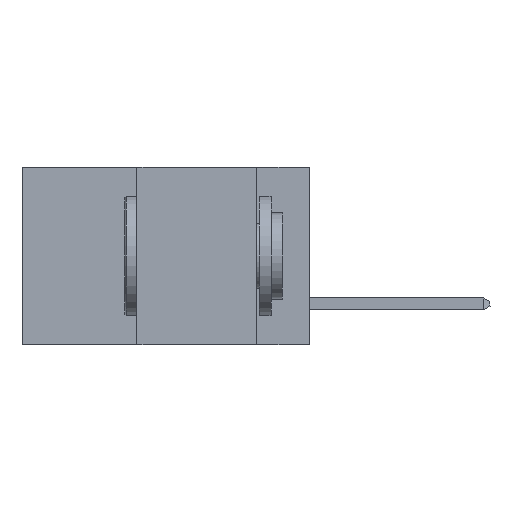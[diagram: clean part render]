
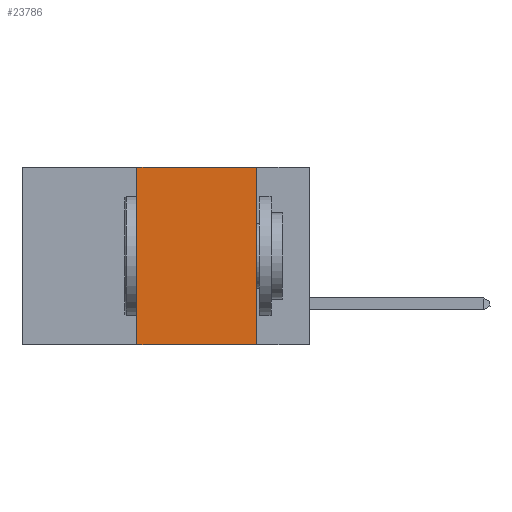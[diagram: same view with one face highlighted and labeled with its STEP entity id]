
A CAD part, left-side view. The second image highlights one B-rep face of the part: STEP entity #23786.
In plain terms, the highlighted planar face has unit normal (-1, 0, 0).
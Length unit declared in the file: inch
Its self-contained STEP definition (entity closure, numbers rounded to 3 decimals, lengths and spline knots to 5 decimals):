
#827 = DIRECTION ( 'NONE',  ( 0., -1., 0. ) ) ;
#1210 = CARTESIAN_POINT ( 'NONE',  ( 0., 0.36, -0.37 ) ) ;
#1501 = VECTOR ( 'NONE', #12696, 39.37008 ) ;
#2147 = VECTOR ( 'NONE', #4223, 39.37008 ) ;
#4177 = VERTEX_POINT ( 'NONE', #1210 ) ;
#4223 = DIRECTION ( 'NONE',  ( 0., 0., 1. ) ) ;
#4787 = CARTESIAN_POINT ( 'NONE',  ( 0., 0.11, 0. ) ) ;
#5059 = CARTESIAN_POINT ( 'NONE',  ( 0., 0.6, -0.37 ) ) ;
#7456 = VERTEX_POINT ( 'NONE', #10748 ) ;
#8641 = DIRECTION ( 'NONE',  ( 1., 0., 0. ) ) ;
#10168 = LINE ( 'NONE', #28794, #1501 ) ;
#10748 = CARTESIAN_POINT ( 'NONE',  ( 0., 0.36, 0. ) ) ;
#12696 = DIRECTION ( 'NONE',  ( 0., 0., -1. ) ) ;
#12841 = EDGE_LOOP ( 'NONE', ( #26368, #26429, #26722, #27407 ) ) ;
#13901 = CARTESIAN_POINT ( 'NONE',  ( 0., 0.36, 0. ) ) ;
#13971 = EDGE_CURVE ( 'NONE', #7456, #37401, #40915, .T. ) ;
#15102 = CARTESIAN_POINT ( 'NONE',  ( 0., 0.11, -0.37 ) ) ;
#15687 = LINE ( 'NONE', #5059, #23296 ) ;
#17340 = AXIS2_PLACEMENT_3D ( 'NONE', #28011, #8641, #31222 ) ;
#21382 = EDGE_CURVE ( 'NONE', #4177, #41673, #15687, .T. ) ;
#21553 = PLANE ( 'NONE',  #17340 ) ;
#22128 = FACE_OUTER_BOUND ( 'NONE', #12841, .T. ) ;
#23296 = VECTOR ( 'NONE', #27714, 39.37008 ) ;
#23786 = ADVANCED_FACE ( 'NONE', ( #22128 ), #21553, .F. ) ;
#26368 = ORIENTED_EDGE ( 'NONE', *, *, #36348, .F. ) ;
#26429 = ORIENTED_EDGE ( 'NONE', *, *, #13971, .F. ) ;
#26722 = ORIENTED_EDGE ( 'NONE', *, *, #34240, .F. ) ;
#27407 = ORIENTED_EDGE ( 'NONE', *, *, #21382, .T. ) ;
#27714 = DIRECTION ( 'NONE',  ( 0., -1., 0. ) ) ;
#28005 = LINE ( 'NONE', #13901, #2147 ) ;
#28011 = CARTESIAN_POINT ( 'NONE',  ( 0., 0.6, 0. ) ) ;
#28794 = CARTESIAN_POINT ( 'NONE',  ( 0., 0.11, 0. ) ) ;
#29872 = CARTESIAN_POINT ( 'NONE',  ( 0., 0.6, 0. ) ) ;
#31222 = DIRECTION ( 'NONE',  ( 0., 0., -1. ) ) ;
#32543 = VECTOR ( 'NONE', #827, 39.37008 ) ;
#34240 = EDGE_CURVE ( 'NONE', #4177, #7456, #28005, .T. ) ;
#36348 = EDGE_CURVE ( 'NONE', #37401, #41673, #10168, .T. ) ;
#37401 = VERTEX_POINT ( 'NONE', #4787 ) ;
#40915 = LINE ( 'NONE', #29872, #32543 ) ;
#41673 = VERTEX_POINT ( 'NONE', #15102 ) ;
